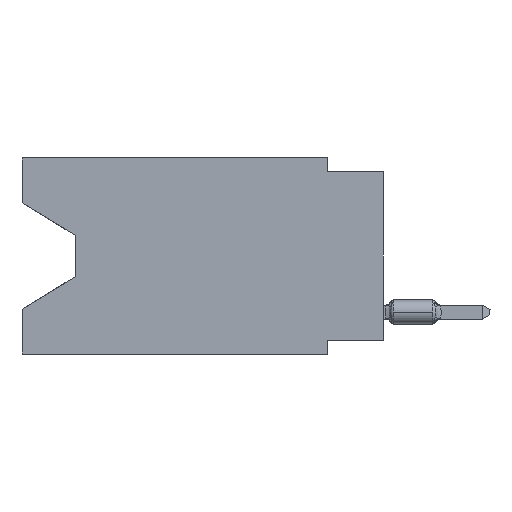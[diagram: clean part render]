
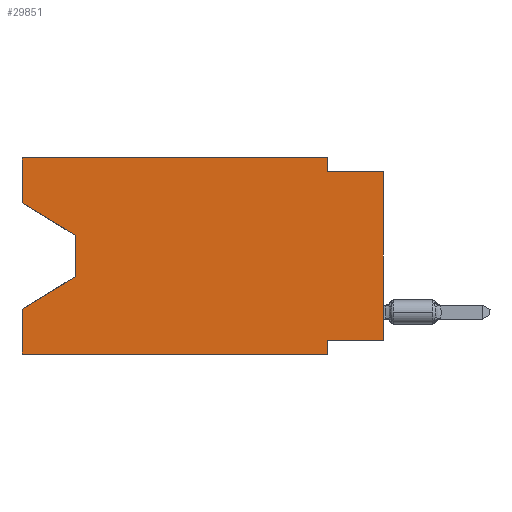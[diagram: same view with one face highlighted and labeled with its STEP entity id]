
A CAD part, left-side view. The second image highlights one B-rep face of the part: STEP entity #29851.
In plain terms, the highlighted planar face has unit normal (-1, 0, 0).
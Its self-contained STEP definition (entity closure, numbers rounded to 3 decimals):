
#68 = VECTOR ( 'NONE', #36343, 1000. ) ;
#1893 = EDGE_CURVE ( 'NONE', #7353, #7450, #42073, .T. ) ;
#2546 = EDGE_CURVE ( 'NONE', #27503, #24127, #5384, .T. ) ;
#4847 = EDGE_CURVE ( 'NONE', #8967, #23385, #10852, .T. ) ;
#5181 = LINE ( 'NONE', #22902, #20280 ) ;
#5333 = EDGE_CURVE ( 'NONE', #41739, #30025, #32308, .T. ) ;
#5384 = LINE ( 'NONE', #22868, #26536 ) ;
#5780 = EDGE_CURVE ( 'NONE', #27503, #17130, #25532, .T. ) ;
#6181 = LINE ( 'NONE', #19880, #28562 ) ;
#6914 = ORIENTED_EDGE ( 'NONE', *, *, #42004, .F. ) ;
#7065 = EDGE_CURVE ( 'NONE', #8967, #27083, #39340, .T. ) ;
#7353 = VERTEX_POINT ( 'NONE', #20445 ) ;
#7450 = VERTEX_POINT ( 'NONE', #28527 ) ;
#8177 = DIRECTION ( 'NONE',  ( 0., -1., 0. ) ) ;
#8967 = VERTEX_POINT ( 'NONE', #40809 ) ;
#10241 = VECTOR ( 'NONE', #8177, 1000. ) ;
#10407 = PLANE ( 'NONE',  #21751 ) ;
#10455 = LINE ( 'NONE', #24171, #25975 ) ;
#10628 = FACE_OUTER_BOUND ( 'NONE', #15218, .T. ) ;
#10852 = LINE ( 'NONE', #17626, #28748 ) ;
#12915 = LINE ( 'NONE', #36965, #26738 ) ;
#13549 = DIRECTION ( 'NONE',  ( 1., 0., 0. ) ) ;
#13824 = VECTOR ( 'NONE', #14657, 1000. ) ;
#14029 = ORIENTED_EDGE ( 'NONE', *, *, #19238, .T. ) ;
#14657 = DIRECTION ( 'NONE',  ( 0., 1., 0. ) ) ;
#15123 = ORIENTED_EDGE ( 'NONE', *, *, #4847, .T. ) ;
#15218 = EDGE_LOOP ( 'NONE', ( #40592, #33271, #14029, #26699, #23696, #37668, #35236, #15123, #27536, #6914, #30219, #37458 ) ) ;
#16037 = CARTESIAN_POINT ( 'NONE',  ( 0., 16.383, -2.038 ) ) ;
#16170 = CARTESIAN_POINT ( 'NONE',  ( 0., 2.54, -8.89 ) ) ;
#17130 = VERTEX_POINT ( 'NONE', #16170 ) ;
#17626 = CARTESIAN_POINT ( 'NONE',  ( 0., 0., 0. ) ) ;
#18744 = CARTESIAN_POINT ( 'NONE',  ( 0., 16.383, -6.852 ) ) ;
#19238 = EDGE_CURVE ( 'NONE', #30025, #24127, #5181, .T. ) ;
#19408 = CARTESIAN_POINT ( 'NONE',  ( 0., 2.54, -0.635 ) ) ;
#19880 = CARTESIAN_POINT ( 'NONE',  ( 0., 2.54, 0. ) ) ;
#20280 = VECTOR ( 'NONE', #22257, 1000. ) ;
#20445 = CARTESIAN_POINT ( 'NONE',  ( 0., 16.383, -2.038 ) ) ;
#21751 = AXIS2_PLACEMENT_3D ( 'NONE', #27262, #13549, #23661 ) ;
#22257 = DIRECTION ( 'NONE',  ( 0., 0.855, -0.519 ) ) ;
#22868 = CARTESIAN_POINT ( 'NONE',  ( 0., 16.383, 0. ) ) ;
#22902 = CARTESIAN_POINT ( 'NONE',  ( 0., 13.97, -5.385 ) ) ;
#23385 = VERTEX_POINT ( 'NONE', #26687 ) ;
#23661 = DIRECTION ( 'NONE',  ( 0., 0., -1. ) ) ;
#23696 = ORIENTED_EDGE ( 'NONE', *, *, #5780, .T. ) ;
#23979 = EDGE_CURVE ( 'NONE', #7450, #24536, #10455, .T. ) ;
#24127 = VERTEX_POINT ( 'NONE', #18744 ) ;
#24171 = CARTESIAN_POINT ( 'NONE',  ( 0., 16.383, 0. ) ) ;
#24209 = CARTESIAN_POINT ( 'NONE',  ( 0., 13.97, -3.505 ) ) ;
#24536 = VERTEX_POINT ( 'NONE', #32633 ) ;
#24569 = DIRECTION ( 'NONE',  ( 0., 0., 1. ) ) ;
#24788 = CARTESIAN_POINT ( 'NONE',  ( 0., 16.383, 0. ) ) ;
#25244 = CARTESIAN_POINT ( 'NONE',  ( 0., 0., -0.635 ) ) ;
#25449 = DIRECTION ( 'NONE',  ( 0., 0., 1. ) ) ;
#25532 = LINE ( 'NONE', #29112, #41728 ) ;
#25975 = VECTOR ( 'NONE', #37859, 1000. ) ;
#26536 = VECTOR ( 'NONE', #43086, 1000. ) ;
#26687 = CARTESIAN_POINT ( 'NONE',  ( 0., 0., -0.635 ) ) ;
#26699 = ORIENTED_EDGE ( 'NONE', *, *, #2546, .F. ) ;
#26738 = VECTOR ( 'NONE', #36730, 1000. ) ;
#27083 = VERTEX_POINT ( 'NONE', #35057 ) ;
#27262 = CARTESIAN_POINT ( 'NONE',  ( 0., 16.383, 0. ) ) ;
#27503 = VERTEX_POINT ( 'NONE', #28632 ) ;
#27536 = ORIENTED_EDGE ( 'NONE', *, *, #31594, .F. ) ;
#27966 = LINE ( 'NONE', #25244, #10241 ) ;
#28527 = CARTESIAN_POINT ( 'NONE',  ( 0., 16.383, 0. ) ) ;
#28562 = VECTOR ( 'NONE', #36954, 1000. ) ;
#28632 = CARTESIAN_POINT ( 'NONE',  ( 0., 16.383, -8.89 ) ) ;
#28748 = VECTOR ( 'NONE', #24569, 1000. ) ;
#29112 = CARTESIAN_POINT ( 'NONE',  ( 0., 16.383, -8.89 ) ) ;
#29358 = EDGE_CURVE ( 'NONE', #27083, #17130, #12915, .T. ) ;
#29728 = DIRECTION ( 'NONE',  ( 0., -0.855, -0.519 ) ) ;
#29819 = EDGE_CURVE ( 'NONE', #7353, #41739, #33097, .T. ) ;
#29851 = ADVANCED_FACE ( 'NONE', ( #10628 ), #10407, .F. ) ;
#30025 = VERTEX_POINT ( 'NONE', #31729 ) ;
#30219 = ORIENTED_EDGE ( 'NONE', *, *, #23979, .F. ) ;
#31594 = EDGE_CURVE ( 'NONE', #38043, #23385, #27966, .T. ) ;
#31729 = CARTESIAN_POINT ( 'NONE',  ( 0., 13.97, -5.385 ) ) ;
#32308 = LINE ( 'NONE', #42407, #68 ) ;
#32633 = CARTESIAN_POINT ( 'NONE',  ( 0., 2.54, 0. ) ) ;
#33097 = LINE ( 'NONE', #16037, #33211 ) ;
#33211 = VECTOR ( 'NONE', #29728, 1000. ) ;
#33271 = ORIENTED_EDGE ( 'NONE', *, *, #5333, .T. ) ;
#35057 = CARTESIAN_POINT ( 'NONE',  ( 0., 2.54, -8.255 ) ) ;
#35108 = CARTESIAN_POINT ( 'NONE',  ( 0., 0., -8.255 ) ) ;
#35236 = ORIENTED_EDGE ( 'NONE', *, *, #7065, .F. ) ;
#36343 = DIRECTION ( 'NONE',  ( 0., 0., -1. ) ) ;
#36730 = DIRECTION ( 'NONE',  ( 0., 0., -1. ) ) ;
#36954 = DIRECTION ( 'NONE',  ( 0., 0., -1. ) ) ;
#36965 = CARTESIAN_POINT ( 'NONE',  ( 0., 2.54, -8.89 ) ) ;
#37458 = ORIENTED_EDGE ( 'NONE', *, *, #1893, .F. ) ;
#37668 = ORIENTED_EDGE ( 'NONE', *, *, #29358, .F. ) ;
#37859 = DIRECTION ( 'NONE',  ( 0., -1., 0. ) ) ;
#38043 = VERTEX_POINT ( 'NONE', #19408 ) ;
#39340 = LINE ( 'NONE', #35108, #13824 ) ;
#40592 = ORIENTED_EDGE ( 'NONE', *, *, #29819, .T. ) ;
#40809 = CARTESIAN_POINT ( 'NONE',  ( 0., 0., -8.255 ) ) ;
#41589 = VECTOR ( 'NONE', #25449, 1000. ) ;
#41728 = VECTOR ( 'NONE', #43232, 1000. ) ;
#41739 = VERTEX_POINT ( 'NONE', #24209 ) ;
#42004 = EDGE_CURVE ( 'NONE', #24536, #38043, #6181, .T. ) ;
#42073 = LINE ( 'NONE', #24788, #41589 ) ;
#42407 = CARTESIAN_POINT ( 'NONE',  ( 0., 13.97, -3.505 ) ) ;
#43086 = DIRECTION ( 'NONE',  ( 0., 0., 1. ) ) ;
#43232 = DIRECTION ( 'NONE',  ( 0., -1., 0. ) ) ;
